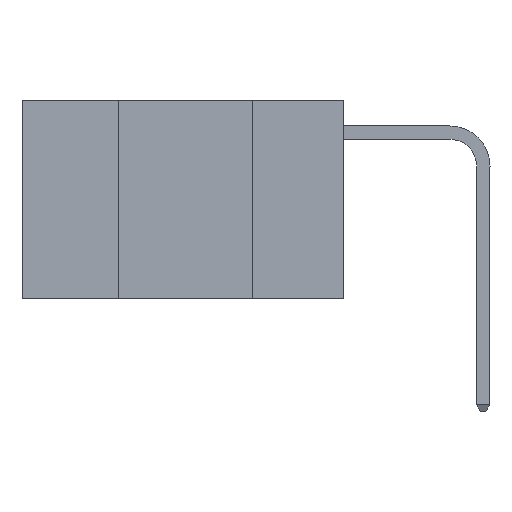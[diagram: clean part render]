
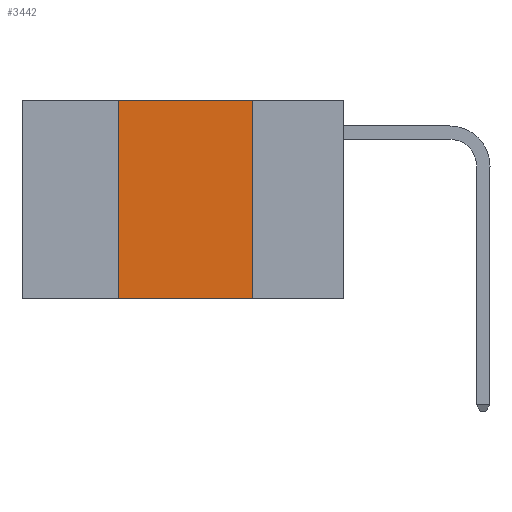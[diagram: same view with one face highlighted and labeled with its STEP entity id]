
A CAD part, left-side view. The second image highlights one B-rep face of the part: STEP entity #3442.
In plain terms, the highlighted planar face has unit normal (-1, 0, 0).
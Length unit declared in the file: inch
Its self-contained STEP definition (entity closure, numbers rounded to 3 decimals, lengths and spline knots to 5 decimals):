
#89 = EDGE_CURVE ( 'NONE', #4188, #19908, #2541, .T. ) ;
#556 = DIRECTION ( 'NONE',  ( 0., 0., -1. ) ) ;
#567 = EDGE_CURVE ( 'NONE', #19908, #8525, #11134, .T. ) ;
#632 = EDGE_CURVE ( 'NONE', #8525, #9224, #13997, .T. ) ;
#1415 = EDGE_LOOP ( 'NONE', ( #5564, #15382, #20822, #10150 ) ) ;
#2541 = LINE ( 'NONE', #15631, #6569 ) ;
#3442 = ADVANCED_FACE ( 'NONE', ( #16009 ), #5611, .F. ) ;
#3975 = CARTESIAN_POINT ( 'NONE',  ( 0., 0.6, 0. ) ) ;
#4036 = CARTESIAN_POINT ( 'NONE',  ( 0., 0.17, 0. ) ) ;
#4188 = VERTEX_POINT ( 'NONE', #14669 ) ;
#5022 = VECTOR ( 'NONE', #6042, 39.37008 ) ;
#5564 = ORIENTED_EDGE ( 'NONE', *, *, #632, .F. ) ;
#5611 = PLANE ( 'NONE',  #14627 ) ;
#5745 = CARTESIAN_POINT ( 'NONE',  ( 0., 0.17, -0.37 ) ) ;
#6042 = DIRECTION ( 'NONE',  ( 0., 0., -1. ) ) ;
#6569 = VECTOR ( 'NONE', #15269, 39.37008 ) ;
#6627 = VECTOR ( 'NONE', #18810, 39.37008 ) ;
#7192 = LINE ( 'NONE', #17621, #11168 ) ;
#8525 = VERTEX_POINT ( 'NONE', #4036 ) ;
#8710 = CARTESIAN_POINT ( 'NONE',  ( 0., 0.42, 0. ) ) ;
#9224 = VERTEX_POINT ( 'NONE', #5745 ) ;
#10150 = ORIENTED_EDGE ( 'NONE', *, *, #10632, .T. ) ;
#10632 = EDGE_CURVE ( 'NONE', #4188, #9224, #7192, .T. ) ;
#10831 = DIRECTION ( 'NONE',  ( 1., 0., 0. ) ) ;
#10979 = DIRECTION ( 'NONE',  ( 0., -1., 0. ) ) ;
#11134 = LINE ( 'NONE', #11224, #6627 ) ;
#11168 = VECTOR ( 'NONE', #10979, 39.37008 ) ;
#11224 = CARTESIAN_POINT ( 'NONE',  ( 0., 0.6, 0. ) ) ;
#13997 = LINE ( 'NONE', #14160, #5022 ) ;
#14160 = CARTESIAN_POINT ( 'NONE',  ( 0., 0.17, 0. ) ) ;
#14627 = AXIS2_PLACEMENT_3D ( 'NONE', #3975, #10831, #556 ) ;
#14669 = CARTESIAN_POINT ( 'NONE',  ( 0., 0.42, -0.37 ) ) ;
#15269 = DIRECTION ( 'NONE',  ( 0., 0., 1. ) ) ;
#15382 = ORIENTED_EDGE ( 'NONE', *, *, #567, .F. ) ;
#15631 = CARTESIAN_POINT ( 'NONE',  ( 0., 0.42, 0. ) ) ;
#16009 = FACE_OUTER_BOUND ( 'NONE', #1415, .T. ) ;
#17621 = CARTESIAN_POINT ( 'NONE',  ( 0., 0.6, -0.37 ) ) ;
#18810 = DIRECTION ( 'NONE',  ( 0., -1., 0. ) ) ;
#19908 = VERTEX_POINT ( 'NONE', #8710 ) ;
#20822 = ORIENTED_EDGE ( 'NONE', *, *, #89, .F. ) ;
